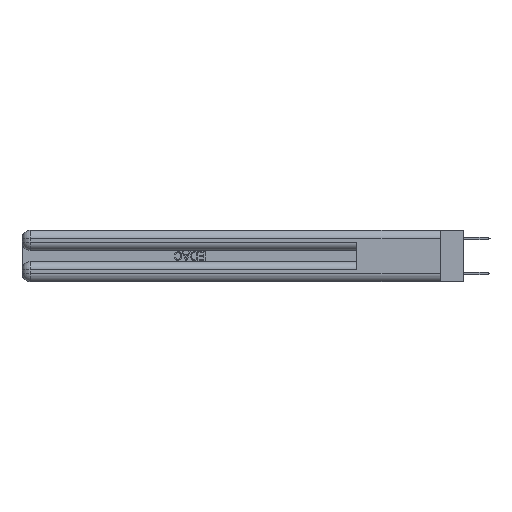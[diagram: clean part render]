
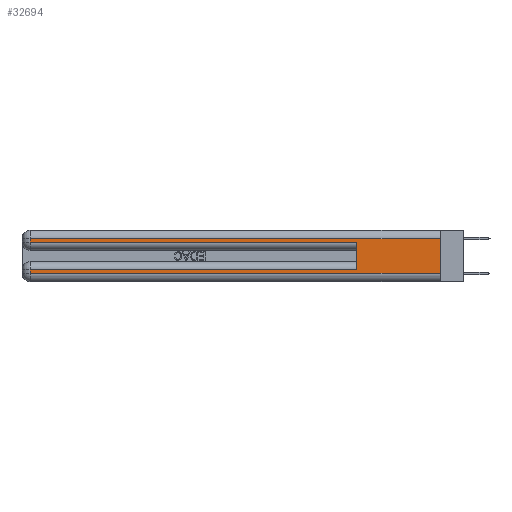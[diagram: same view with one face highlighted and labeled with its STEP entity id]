
A CAD part, left-side view. The second image highlights one B-rep face of the part: STEP entity #32694.
In plain terms, the highlighted planar face has unit normal (-1, 0, 0).
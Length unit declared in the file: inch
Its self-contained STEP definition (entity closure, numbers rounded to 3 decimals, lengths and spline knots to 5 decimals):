
#376 = LINE ( 'NONE', #23445, #17586 ) ;
#397 = VECTOR ( 'NONE', #19041, 39.37008 ) ;
#709 = DIRECTION ( 'NONE',  ( 0., 0., -1. ) ) ;
#1420 = PLANE ( 'NONE',  #17420 ) ;
#2084 = LINE ( 'NONE', #9237, #5545 ) ;
#2311 = CARTESIAN_POINT ( 'NONE',  ( 0., 2.94, 0.085 ) ) ;
#2987 = CARTESIAN_POINT ( 'NONE',  ( 0., 0., 0.31 ) ) ;
#3044 = EDGE_CURVE ( 'NONE', #3819, #28668, #11565, .T. ) ;
#3581 = DIRECTION ( 'NONE',  ( 0., 0., -1. ) ) ;
#3587 = DIRECTION ( 'NONE',  ( 0., 1., 0. ) ) ;
#3819 = VERTEX_POINT ( 'NONE', #12434 ) ;
#4239 = FACE_OUTER_BOUND ( 'NONE', #32731, .T. ) ;
#5545 = VECTOR ( 'NONE', #11717, 39.37008 ) ;
#5619 = EDGE_CURVE ( 'NONE', #13805, #23915, #31632, .T. ) ;
#5643 = EDGE_CURVE ( 'NONE', #15580, #25865, #10618, .T. ) ;
#5735 = CARTESIAN_POINT ( 'NONE',  ( 0., 0.6, 0.085 ) ) ;
#5839 = VECTOR ( 'NONE', #13190, 39.37008 ) ;
#6453 = DIRECTION ( 'NONE',  ( 0., 0., -1. ) ) ;
#6626 = ORIENTED_EDGE ( 'NONE', *, *, #26152, .T. ) ;
#8738 = DIRECTION ( 'NONE',  ( 0., 1., 0. ) ) ;
#8760 = CARTESIAN_POINT ( 'NONE',  ( 0., 0., 0.285 ) ) ;
#9069 = EDGE_CURVE ( 'NONE', #13805, #28668, #14929, .T. ) ;
#9138 = VECTOR ( 'NONE', #25066, 39.37008 ) ;
#9237 = CARTESIAN_POINT ( 'NONE',  ( 0., 0., 0.37 ) ) ;
#9780 = ORIENTED_EDGE ( 'NONE', *, *, #24572, .T. ) ;
#10618 = LINE ( 'NONE', #2987, #30326 ) ;
#11565 = LINE ( 'NONE', #8760, #397 ) ;
#11717 = DIRECTION ( 'NONE',  ( 0., 0., -1. ) ) ;
#11893 = CARTESIAN_POINT ( 'NONE',  ( 0., 0.6, 0.285 ) ) ;
#12378 = EDGE_CURVE ( 'NONE', #15580, #24069, #2084, .T. ) ;
#12434 = CARTESIAN_POINT ( 'NONE',  ( 0., 2.94, 0.285 ) ) ;
#13190 = DIRECTION ( 'NONE',  ( 0., -1., 0. ) ) ;
#13805 = VERTEX_POINT ( 'NONE', #5735 ) ;
#14929 = LINE ( 'NONE', #17929, #9138 ) ;
#15232 = CARTESIAN_POINT ( 'NONE',  ( 0., 2.94, 0.31 ) ) ;
#15580 = VERTEX_POINT ( 'NONE', #23137 ) ;
#16445 = ORIENTED_EDGE ( 'NONE', *, *, #3044, .T. ) ;
#16585 = LINE ( 'NONE', #21572, #18664 ) ;
#17420 = AXIS2_PLACEMENT_3D ( 'NONE', #26817, #21336, #3581 ) ;
#17586 = VECTOR ( 'NONE', #709, 39.37008 ) ;
#17756 = CARTESIAN_POINT ( 'NONE',  ( 0., 0., 0.085 ) ) ;
#17929 = CARTESIAN_POINT ( 'NONE',  ( 0., 0.6, 0.145 ) ) ;
#18543 = VECTOR ( 'NONE', #3587, 39.37008 ) ;
#18664 = VECTOR ( 'NONE', #6453, 39.37008 ) ;
#19041 = DIRECTION ( 'NONE',  ( 0., -1., 0. ) ) ;
#19712 = CARTESIAN_POINT ( 'NONE',  ( 0., 2.94, 0.06 ) ) ;
#19745 = VERTEX_POINT ( 'NONE', #19712 ) ;
#20146 = ORIENTED_EDGE ( 'NONE', *, *, #12378, .F. ) ;
#21336 = DIRECTION ( 'NONE',  ( 1., 0., 0. ) ) ;
#21572 = CARTESIAN_POINT ( 'NONE',  ( 0., 2.94, 0.37 ) ) ;
#22665 = ORIENTED_EDGE ( 'NONE', *, *, #5643, .T. ) ;
#23137 = CARTESIAN_POINT ( 'NONE',  ( 0., 0., 0.31 ) ) ;
#23445 = CARTESIAN_POINT ( 'NONE',  ( 0., 2.94, 0.37 ) ) ;
#23915 = VERTEX_POINT ( 'NONE', #2311 ) ;
#24069 = VERTEX_POINT ( 'NONE', #27108 ) ;
#24572 = EDGE_CURVE ( 'NONE', #19745, #24069, #25490, .T. ) ;
#25066 = DIRECTION ( 'NONE',  ( 0., 0., 1. ) ) ;
#25267 = ORIENTED_EDGE ( 'NONE', *, *, #9069, .F. ) ;
#25490 = LINE ( 'NONE', #26130, #5839 ) ;
#25865 = VERTEX_POINT ( 'NONE', #15232 ) ;
#26130 = CARTESIAN_POINT ( 'NONE',  ( 0., 0., 0.06 ) ) ;
#26152 = EDGE_CURVE ( 'NONE', #25865, #3819, #376, .T. ) ;
#26232 = ORIENTED_EDGE ( 'NONE', *, *, #5619, .T. ) ;
#26792 = EDGE_CURVE ( 'NONE', #23915, #19745, #16585, .T. ) ;
#26817 = CARTESIAN_POINT ( 'NONE',  ( 0., 0., 0.37 ) ) ;
#27108 = CARTESIAN_POINT ( 'NONE',  ( 0., 0., 0.06 ) ) ;
#28668 = VERTEX_POINT ( 'NONE', #11893 ) ;
#29120 = ORIENTED_EDGE ( 'NONE', *, *, #26792, .T. ) ;
#30326 = VECTOR ( 'NONE', #8738, 39.37008 ) ;
#31632 = LINE ( 'NONE', #17756, #18543 ) ;
#32694 = ADVANCED_FACE ( 'NONE', ( #4239 ), #1420, .F. ) ;
#32731 = EDGE_LOOP ( 'NONE', ( #20146, #22665, #6626, #16445, #25267, #26232, #29120, #9780 ) ) ;
